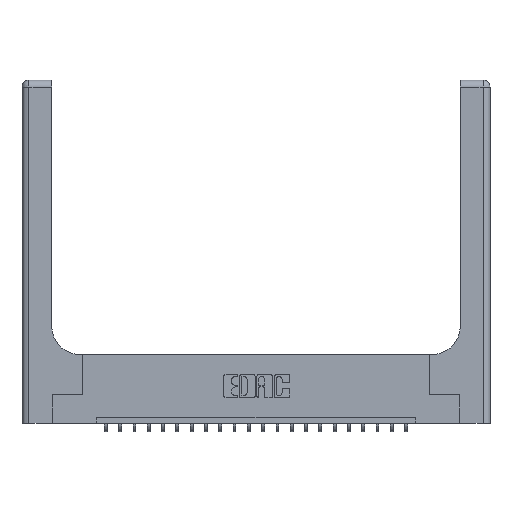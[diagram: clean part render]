
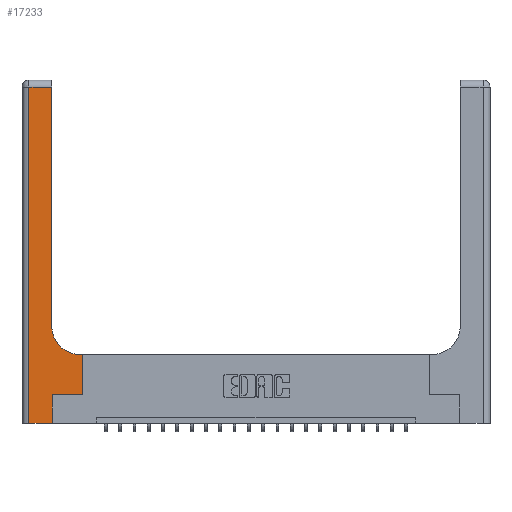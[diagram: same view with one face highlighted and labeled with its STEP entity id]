
A CAD part, top view. The second image highlights one B-rep face of the part: STEP entity #17233.
In plain terms, the highlighted planar face has unit normal (0, 0, 1).
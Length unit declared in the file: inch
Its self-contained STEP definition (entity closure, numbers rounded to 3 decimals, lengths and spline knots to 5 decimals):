
#51 = CARTESIAN_POINT ( 'NONE',  ( 0.528, 0.25, 0.37 ) ) ;
#333 = VERTEX_POINT ( 'NONE', #16738 ) ;
#1508 = EDGE_CURVE ( 'NONE', #16609, #7020, #7246, .T. ) ;
#2165 = LINE ( 'NONE', #20500, #17851 ) ;
#2182 = EDGE_CURVE ( 'NONE', #6855, #16609, #7475, .T. ) ;
#2450 = VERTEX_POINT ( 'NONE', #4069 ) ;
#2659 = VERTEX_POINT ( 'NONE', #5776 ) ;
#3085 = CARTESIAN_POINT ( 'NONE',  ( 0.26, 0.6, 0.37 ) ) ;
#3267 = ORIENTED_EDGE ( 'NONE', *, *, #1508, .T. ) ;
#3313 = VECTOR ( 'NONE', #4736, 39.37008 ) ;
#3320 = DIRECTION ( 'NONE',  ( -1., 0., 0. ) ) ;
#4069 = CARTESIAN_POINT ( 'NONE',  ( 0.06, 2.94, 0.37 ) ) ;
#4105 = EDGE_CURVE ( 'NONE', #7020, #10819, #17614, .T. ) ;
#4263 = EDGE_CURVE ( 'NONE', #333, #2450, #14498, .T. ) ;
#4544 = VERTEX_POINT ( 'NONE', #7945 ) ;
#4736 = DIRECTION ( 'NONE',  ( 0., 1., 0. ) ) ;
#4986 = DIRECTION ( 'NONE',  ( 0., 0., -1. ) ) ;
#5598 = VECTOR ( 'NONE', #15810, 39.37008 ) ;
#5776 = CARTESIAN_POINT ( 'NONE',  ( 0.265, 0., 0.37 ) ) ;
#5804 = CARTESIAN_POINT ( 'NONE',  ( 0., 0., 0.37 ) ) ;
#6043 = VECTOR ( 'NONE', #6581, 39.37008 ) ;
#6316 = AXIS2_PLACEMENT_3D ( 'NONE', #8270, #13325, #3320 ) ;
#6420 = CARTESIAN_POINT ( 'NONE',  ( 0.265, 0., 0.37 ) ) ;
#6456 = DIRECTION ( 'NONE',  ( -1., 0., 0. ) ) ;
#6581 = DIRECTION ( 'NONE',  ( 1., 0., 0. ) ) ;
#6855 = VERTEX_POINT ( 'NONE', #11605 ) ;
#7009 = LINE ( 'NONE', #17647, #19254 ) ;
#7020 = VERTEX_POINT ( 'NONE', #10257 ) ;
#7219 = LINE ( 'NONE', #6420, #3313 ) ;
#7246 = LINE ( 'NONE', #3085, #15614 ) ;
#7384 = CARTESIAN_POINT ( 'NONE',  ( 0.06, 0., 0.37 ) ) ;
#7475 = LINE ( 'NONE', #51, #20256 ) ;
#7694 = ORIENTED_EDGE ( 'NONE', *, *, #4105, .T. ) ;
#7945 = CARTESIAN_POINT ( 'NONE',  ( 0.265, 0.25, 0.37 ) ) ;
#8270 = CARTESIAN_POINT ( 'NONE',  ( 0., 3., 0.37 ) ) ;
#8719 = ORIENTED_EDGE ( 'NONE', *, *, #10718, .T. ) ;
#9773 = ORIENTED_EDGE ( 'NONE', *, *, #13992, .T. ) ;
#9945 = LINE ( 'NONE', #16595, #6043 ) ;
#10257 = CARTESIAN_POINT ( 'NONE',  ( 0.51, 0.6, 0.37 ) ) ;
#10718 = EDGE_CURVE ( 'NONE', #10819, #333, #2165, .T. ) ;
#10780 = VERTEX_POINT ( 'NONE', #7384 ) ;
#10819 = VERTEX_POINT ( 'NONE', #15797 ) ;
#11357 = ORIENTED_EDGE ( 'NONE', *, *, #18726, .T. ) ;
#11557 = AXIS2_PLACEMENT_3D ( 'NONE', #14991, #4986, #16686 ) ;
#11605 = CARTESIAN_POINT ( 'NONE',  ( 0.528, 0.25, 0.37 ) ) ;
#12216 = DIRECTION ( 'NONE',  ( 0., 1., 0. ) ) ;
#13181 = ORIENTED_EDGE ( 'NONE', *, *, #4263, .T. ) ;
#13325 = DIRECTION ( 'NONE',  ( 0., 0., -1. ) ) ;
#13371 = DIRECTION ( 'NONE',  ( 0., 1., 0. ) ) ;
#13992 = EDGE_CURVE ( 'NONE', #2450, #10780, #7009, .T. ) ;
#14382 = DIRECTION ( 'NONE',  ( 0., -1., 0. ) ) ;
#14498 = LINE ( 'NONE', #17017, #18370 ) ;
#14743 = CARTESIAN_POINT ( 'NONE',  ( 0.528, 0.6, 0.37 ) ) ;
#14991 = CARTESIAN_POINT ( 'NONE',  ( 0.51, 0.85, 0.37 ) ) ;
#15533 = LINE ( 'NONE', #5804, #5598 ) ;
#15536 = ORIENTED_EDGE ( 'NONE', *, *, #2182, .T. ) ;
#15614 = VECTOR ( 'NONE', #6456, 39.37008 ) ;
#15797 = CARTESIAN_POINT ( 'NONE',  ( 0.26, 0.85, 0.37 ) ) ;
#15810 = DIRECTION ( 'NONE',  ( 1., 0., 0. ) ) ;
#15816 = EDGE_CURVE ( 'NONE', #2659, #4544, #7219, .T. ) ;
#16595 = CARTESIAN_POINT ( 'NONE',  ( 0.265, 0.25, 0.37 ) ) ;
#16609 = VERTEX_POINT ( 'NONE', #14743 ) ;
#16686 = DIRECTION ( 'NONE',  ( 1., 0., 0. ) ) ;
#16738 = CARTESIAN_POINT ( 'NONE',  ( 0.26, 2.94, 0.37 ) ) ;
#17017 = CARTESIAN_POINT ( 'NONE',  ( 0., 2.94, 0.37 ) ) ;
#17233 = ADVANCED_FACE ( 'NONE', ( #19495 ), #21605, .F. ) ;
#17614 = CIRCLE ( 'NONE', #11557, 0.25 ) ;
#17647 = CARTESIAN_POINT ( 'NONE',  ( 0.06, 3., 0.37 ) ) ;
#17851 = VECTOR ( 'NONE', #12216, 39.37008 ) ;
#18137 = EDGE_LOOP ( 'NONE', ( #8719, #13181, #9773, #11357, #21244, #18378, #15536, #3267, #7694 ) ) ;
#18370 = VECTOR ( 'NONE', #20348, 39.37008 ) ;
#18378 = ORIENTED_EDGE ( 'NONE', *, *, #20913, .T. ) ;
#18726 = EDGE_CURVE ( 'NONE', #10780, #2659, #15533, .T. ) ;
#19254 = VECTOR ( 'NONE', #14382, 39.37008 ) ;
#19495 = FACE_OUTER_BOUND ( 'NONE', #18137, .T. ) ;
#20256 = VECTOR ( 'NONE', #13371, 39.37008 ) ;
#20348 = DIRECTION ( 'NONE',  ( -1., 0., 0. ) ) ;
#20500 = CARTESIAN_POINT ( 'NONE',  ( 0.26, 3., 0.37 ) ) ;
#20913 = EDGE_CURVE ( 'NONE', #4544, #6855, #9945, .T. ) ;
#21244 = ORIENTED_EDGE ( 'NONE', *, *, #15816, .T. ) ;
#21605 = PLANE ( 'NONE',  #6316 ) ;
